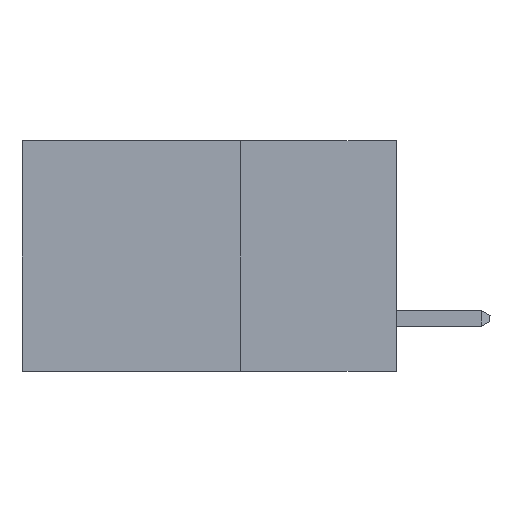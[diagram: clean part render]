
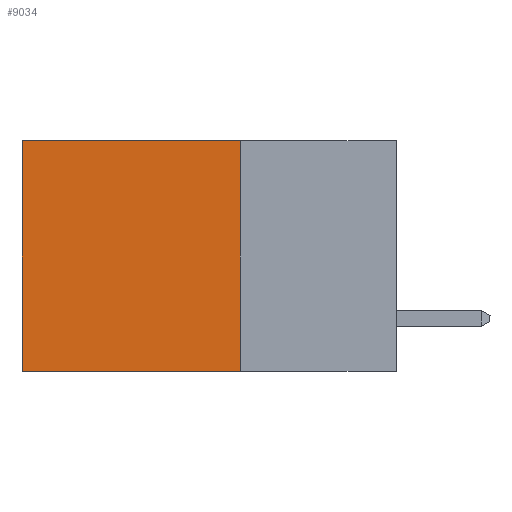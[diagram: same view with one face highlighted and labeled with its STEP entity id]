
A CAD part, left-side view. The second image highlights one B-rep face of the part: STEP entity #9034.
In plain terms, the highlighted planar face has unit normal (-1, 0, 0).
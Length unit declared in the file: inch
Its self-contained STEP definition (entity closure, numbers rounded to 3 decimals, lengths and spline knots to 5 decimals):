
#1098 = LINE ( 'NONE', #8539, #6872 ) ;
#3339 = ORIENTED_EDGE ( 'NONE', *, *, #5452, .F. ) ;
#3413 = VECTOR ( 'NONE', #11940, 39.37008 ) ;
#3424 = ORIENTED_EDGE ( 'NONE', *, *, #4845, .F. ) ;
#3766 = CARTESIAN_POINT ( 'NONE',  ( 0.2615, 0.6, -0.37 ) ) ;
#3834 = EDGE_CURVE ( 'NONE', #7403, #11659, #4421, .T. ) ;
#3915 = PLANE ( 'NONE',  #9889 ) ;
#4406 = LINE ( 'NONE', #16094, #14907 ) ;
#4421 = LINE ( 'NONE', #13274, #3413 ) ;
#4629 = DIRECTION ( 'NONE',  ( 0., 0., -1. ) ) ;
#4786 = VECTOR ( 'NONE', #15565, 39.37008 ) ;
#4845 = EDGE_CURVE ( 'NONE', #7403, #16418, #1098, .T. ) ;
#5096 = DIRECTION ( 'NONE',  ( 1., 0., 0. ) ) ;
#5452 = EDGE_CURVE ( 'NONE', #16418, #8353, #4406, .T. ) ;
#5904 = CARTESIAN_POINT ( 'NONE',  ( 0.2615, 0.25, -0.37 ) ) ;
#6623 = EDGE_CURVE ( 'NONE', #11659, #8353, #7790, .T. ) ;
#6872 = VECTOR ( 'NONE', #4629, 39.37008 ) ;
#7403 = VERTEX_POINT ( 'NONE', #16367 ) ;
#7790 = LINE ( 'NONE', #8029, #4786 ) ;
#8029 = CARTESIAN_POINT ( 'NONE',  ( 0.2615, 0.6, -0.37 ) ) ;
#8353 = VERTEX_POINT ( 'NONE', #3766 ) ;
#8539 = CARTESIAN_POINT ( 'NONE',  ( 0.2615, 0.25, -0.37 ) ) ;
#8992 = CARTESIAN_POINT ( 'NONE',  ( 0.2615, 0.25, -0.37 ) ) ;
#9034 = ADVANCED_FACE ( 'NONE', ( #15376 ), #3915, .F. ) ;
#9889 = AXIS2_PLACEMENT_3D ( 'NONE', #8992, #5096, #14044 ) ;
#11659 = VERTEX_POINT ( 'NONE', #15197 ) ;
#11682 = ORIENTED_EDGE ( 'NONE', *, *, #3834, .T. ) ;
#11940 = DIRECTION ( 'NONE',  ( 0., 1., 0. ) ) ;
#12164 = DIRECTION ( 'NONE',  ( 0., 1., 0. ) ) ;
#13274 = CARTESIAN_POINT ( 'NONE',  ( 0.2615, 0.25, 0. ) ) ;
#14044 = DIRECTION ( 'NONE',  ( 0., 0., -1. ) ) ;
#14907 = VECTOR ( 'NONE', #12164, 39.37008 ) ;
#15197 = CARTESIAN_POINT ( 'NONE',  ( 0.2615, 0.6, 0. ) ) ;
#15376 = FACE_OUTER_BOUND ( 'NONE', #16345, .T. ) ;
#15565 = DIRECTION ( 'NONE',  ( 0., 0., -1. ) ) ;
#16078 = ORIENTED_EDGE ( 'NONE', *, *, #6623, .T. ) ;
#16094 = CARTESIAN_POINT ( 'NONE',  ( 0.2615, 0.25, -0.37 ) ) ;
#16345 = EDGE_LOOP ( 'NONE', ( #16078, #3339, #3424, #11682 ) ) ;
#16367 = CARTESIAN_POINT ( 'NONE',  ( 0.2615, 0.25, 0. ) ) ;
#16418 = VERTEX_POINT ( 'NONE', #5904 ) ;
